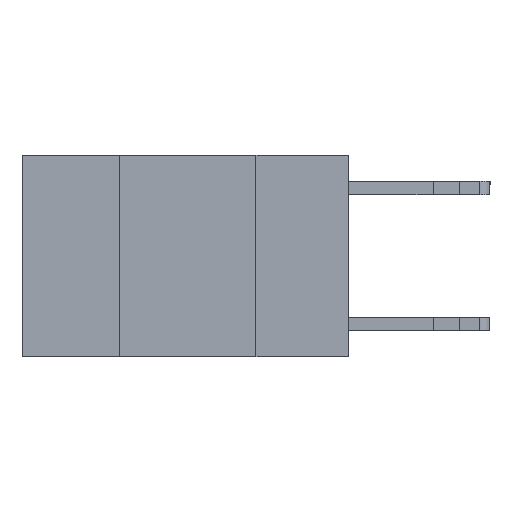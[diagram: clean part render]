
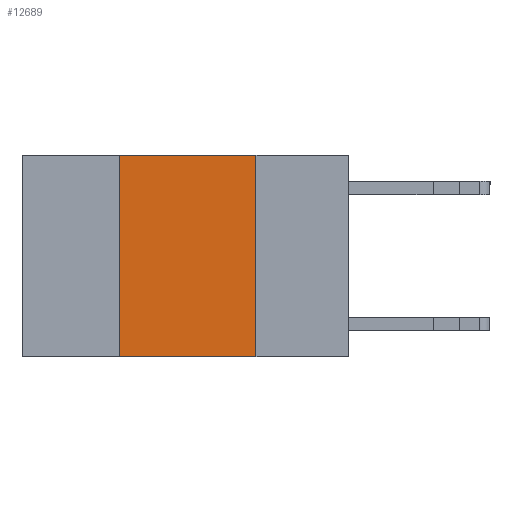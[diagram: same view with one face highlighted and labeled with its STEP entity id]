
A CAD part, left-side view. The second image highlights one B-rep face of the part: STEP entity #12689.
In plain terms, the highlighted planar face has unit normal (-1, 0, 0).
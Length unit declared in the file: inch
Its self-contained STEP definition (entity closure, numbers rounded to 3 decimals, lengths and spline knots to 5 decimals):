
#464 = CARTESIAN_POINT ( 'NONE',  ( 0., 0.6, 0. ) ) ;
#1360 = VERTEX_POINT ( 'NONE', #3787 ) ;
#1406 = LINE ( 'NONE', #464, #12781 ) ;
#1781 = VERTEX_POINT ( 'NONE', #2767 ) ;
#2767 = CARTESIAN_POINT ( 'NONE',  ( 0., 0.42, 0. ) ) ;
#3227 = DIRECTION ( 'NONE',  ( 0., -1., 0. ) ) ;
#3244 = DIRECTION ( 'NONE',  ( 1., 0., 0. ) ) ;
#3787 = CARTESIAN_POINT ( 'NONE',  ( 0., 0.17, -0.37 ) ) ;
#4088 = LINE ( 'NONE', #12931, #8685 ) ;
#4123 = EDGE_CURVE ( 'NONE', #1781, #6595, #1406, .T. ) ;
#4158 = LINE ( 'NONE', #12336, #11424 ) ;
#4230 = PLANE ( 'NONE',  #7041 ) ;
#4509 = DIRECTION ( 'NONE',  ( 0., -1., 0. ) ) ;
#4673 = EDGE_CURVE ( 'NONE', #11417, #1781, #11083, .T. ) ;
#5949 = DIRECTION ( 'NONE',  ( 0., 0., 1. ) ) ;
#6595 = VERTEX_POINT ( 'NONE', #10088 ) ;
#6627 = VECTOR ( 'NONE', #5949, 39.37008 ) ;
#7041 = AXIS2_PLACEMENT_3D ( 'NONE', #8286, #3244, #11347 ) ;
#7410 = ORIENTED_EDGE ( 'NONE', *, *, #9968, .T. ) ;
#8286 = CARTESIAN_POINT ( 'NONE',  ( 0., 0.6, 0. ) ) ;
#8685 = VECTOR ( 'NONE', #10061, 39.37008 ) ;
#8938 = ORIENTED_EDGE ( 'NONE', *, *, #4673, .F. ) ;
#9263 = EDGE_LOOP ( 'NONE', ( #12480, #12170, #8938, #7410 ) ) ;
#9466 = CARTESIAN_POINT ( 'NONE',  ( 0., 0.42, -0.37 ) ) ;
#9968 = EDGE_CURVE ( 'NONE', #11417, #1360, #4158, .T. ) ;
#10061 = DIRECTION ( 'NONE',  ( 0., 0., -1. ) ) ;
#10088 = CARTESIAN_POINT ( 'NONE',  ( 0., 0.17, 0. ) ) ;
#10265 = CARTESIAN_POINT ( 'NONE',  ( 0., 0.42, 0. ) ) ;
#11083 = LINE ( 'NONE', #10265, #6627 ) ;
#11347 = DIRECTION ( 'NONE',  ( 0., 0., -1. ) ) ;
#11417 = VERTEX_POINT ( 'NONE', #9466 ) ;
#11424 = VECTOR ( 'NONE', #3227, 39.37008 ) ;
#11609 = EDGE_CURVE ( 'NONE', #6595, #1360, #4088, .T. ) ;
#12170 = ORIENTED_EDGE ( 'NONE', *, *, #4123, .F. ) ;
#12336 = CARTESIAN_POINT ( 'NONE',  ( 0., 0.6, -0.37 ) ) ;
#12429 = FACE_OUTER_BOUND ( 'NONE', #9263, .T. ) ;
#12480 = ORIENTED_EDGE ( 'NONE', *, *, #11609, .F. ) ;
#12689 = ADVANCED_FACE ( 'NONE', ( #12429 ), #4230, .F. ) ;
#12781 = VECTOR ( 'NONE', #4509, 39.37008 ) ;
#12931 = CARTESIAN_POINT ( 'NONE',  ( 0., 0.17, 0. ) ) ;
